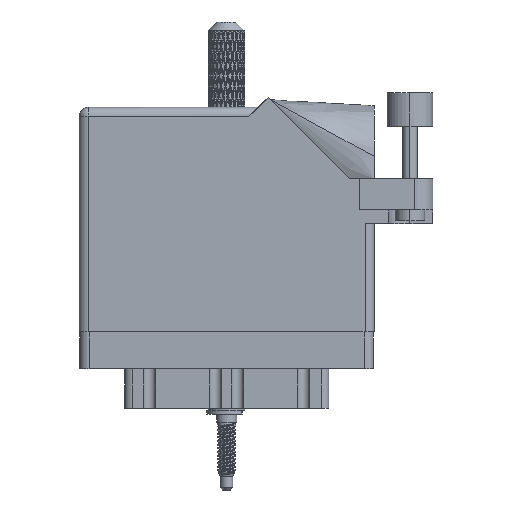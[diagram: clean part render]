
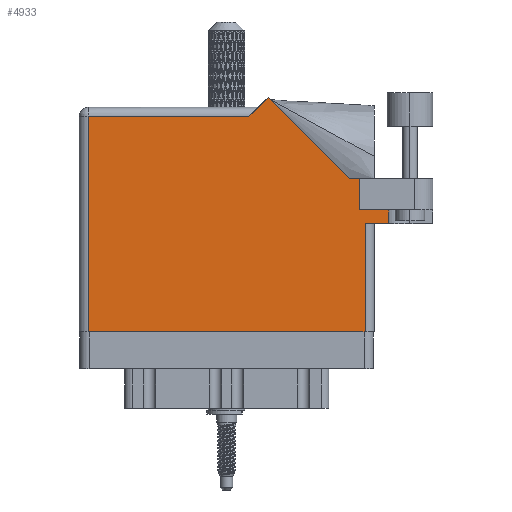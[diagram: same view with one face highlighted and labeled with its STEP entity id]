
A CAD part, front view. The second image highlights one B-rep face of the part: STEP entity #4933.
In plain terms, the highlighted face is planar.
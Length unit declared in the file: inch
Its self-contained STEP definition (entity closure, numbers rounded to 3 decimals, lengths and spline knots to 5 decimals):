
#2073 = CARTESIAN_POINT ( 'NONE',  ( 0., 1.468, 0. ) ) ;
#2655 = VECTOR ( 'NONE', #67782, 39.37008 ) ;
#2757 = CARTESIAN_POINT ( 'NONE',  ( 0.062, 1.468, 0. ) ) ;
#2888 = LINE ( 'NONE', #51669, #55897 ) ;
#3194 = CARTESIAN_POINT ( 'NONE',  ( 1.28771, 1.60071, 0. ) ) ;
#3305 = ORIENTED_EDGE ( 'NONE', *, *, #72947, .T. ) ;
#4055 = DIRECTION ( 'NONE',  ( 1., 0., 0. ) ) ;
#4379 = VECTOR ( 'NONE', #51262, 39.37008 ) ;
#4933 = ADVANCED_FACE ( 'NONE', ( #61687 ), #69104, .F. ) ;
#5165 = ORIENTED_EDGE ( 'NONE', *, *, #74992, .F. ) ;
#5422 = VERTEX_POINT ( 'NONE', #87947 ) ;
#8835 = ORIENTED_EDGE ( 'NONE', *, *, #32671, .F. ) ;
#10510 = EDGE_CURVE ( 'NONE', #98505, #39242, #65467, .T. ) ;
#13570 = CARTESIAN_POINT ( 'NONE',  ( 1.91, 0.831, 0. ) ) ;
#14255 = EDGE_CURVE ( 'NONE', #56066, #93212, #92200, .T. ) ;
#14977 = CARTESIAN_POINT ( 'NONE',  ( 1.948, 0., 0. ) ) ;
#15754 = CARTESIAN_POINT ( 'NONE',  ( 0.062, 0., 0. ) ) ;
#16635 = CARTESIAN_POINT ( 'NONE',  ( 2.1115, 0.831, 0. ) ) ;
#18187 = DIRECTION ( 'NONE',  ( 0., 1., 0. ) ) ;
#18232 = DIRECTION ( 'NONE',  ( 1., 0., 0. ) ) ;
#18774 = ORIENTED_EDGE ( 'NONE', *, *, #67635, .T. ) ;
#19482 = VECTOR ( 'NONE', #30221, 39.37008 ) ;
#20450 = CARTESIAN_POINT ( 'NONE',  ( 2.41, 1.044, 0. ) ) ;
#21317 = VECTOR ( 'NONE', #47770, 39.37008 ) ;
#22718 = ORIENTED_EDGE ( 'NONE', *, *, #14255, .T. ) ;
#23442 = CARTESIAN_POINT ( 'NONE',  ( 1.948, 0.737, 0. ) ) ;
#27198 = LINE ( 'NONE', #104330, #74530 ) ;
#27786 = VERTEX_POINT ( 'NONE', #16635 ) ;
#29893 = VERTEX_POINT ( 'NONE', #14977 ) ;
#30221 = DIRECTION ( 'NONE',  ( -0.707, -0.707, 0. ) ) ;
#32671 = EDGE_CURVE ( 'NONE', #27786, #39242, #2888, .T. ) ;
#33191 = VECTOR ( 'NONE', #87369, 39.37008 ) ;
#38700 = VERTEX_POINT ( 'NONE', #52278 ) ;
#39242 = VERTEX_POINT ( 'NONE', #104354 ) ;
#44265 = DIRECTION ( 'NONE',  ( 0., -1., 0. ) ) ;
#45303 = ORIENTED_EDGE ( 'NONE', *, *, #71131, .T. ) ;
#45427 = DIRECTION ( 'NONE',  ( 1., 0., 0. ) ) ;
#45730 = ORIENTED_EDGE ( 'NONE', *, *, #55389, .T. ) ;
#46623 = VECTOR ( 'NONE', #94030, 39.37008 ) ;
#47770 = DIRECTION ( 'NONE',  ( -0.707, 0.707, 0. ) ) ;
#47938 = EDGE_LOOP ( 'NONE', ( #18774, #45730, #48015, #8835, #5165, #84794, #3305, #103992, #45303, #22718, #99225 ) ) ;
#48015 = ORIENTED_EDGE ( 'NONE', *, *, #10510, .T. ) ;
#51262 = DIRECTION ( 'NONE',  ( -1., 0., 0. ) ) ;
#51669 = CARTESIAN_POINT ( 'NONE',  ( 2.1115, 1.16177, 0. ) ) ;
#52278 = CARTESIAN_POINT ( 'NONE',  ( 1.91, 0.831, 0. ) ) ;
#53980 = AXIS2_PLACEMENT_3D ( 'NONE', #101464, #61173, #63257 ) ;
#54621 = VECTOR ( 'NONE', #18232, 39.37008 ) ;
#55389 = EDGE_CURVE ( 'NONE', #29893, #98505, #63235, .T. ) ;
#55696 = LINE ( 'NONE', #64160, #21317 ) ;
#55897 = VECTOR ( 'NONE', #44265, 39.37008 ) ;
#56066 = VERTEX_POINT ( 'NONE', #85608 ) ;
#57472 = EDGE_CURVE ( 'NONE', #93212, #77820, #88430, .T. ) ;
#59547 = CARTESIAN_POINT ( 'NONE',  ( 1.217, 1.53, 0. ) ) ;
#61173 = DIRECTION ( 'NONE',  ( 0., 0., -1. ) ) ;
#61687 = FACE_OUTER_BOUND ( 'NONE', #47938, .T. ) ;
#63235 = LINE ( 'NONE', #23442, #46623 ) ;
#63257 = DIRECTION ( 'NONE',  ( -1., 0., 0. ) ) ;
#64160 = CARTESIAN_POINT ( 'NONE',  ( 1.84442, 1.044, 0. ) ) ;
#65467 = LINE ( 'NONE', #89890, #54621 ) ;
#67635 = EDGE_CURVE ( 'NONE', #77820, #29893, #68750, .T. ) ;
#67679 = CARTESIAN_POINT ( 'NONE',  ( 1.91, 1.044, 0. ) ) ;
#67782 = DIRECTION ( 'NONE',  ( -1., 0., 0. ) ) ;
#68750 = LINE ( 'NONE', #83107, #70322 ) ;
#69104 = PLANE ( 'NONE',  #53980 ) ;
#70111 = VERTEX_POINT ( 'NONE', #3194 ) ;
#70116 = CARTESIAN_POINT ( 'NONE',  ( 1.948, 0.737, 0. ) ) ;
#70322 = VECTOR ( 'NONE', #4055, 39.37008 ) ;
#71131 = EDGE_CURVE ( 'NONE', #70111, #56066, #100910, .T. ) ;
#72493 = EDGE_CURVE ( 'NONE', #5422, #70111, #55696, .T. ) ;
#72947 = EDGE_CURVE ( 'NONE', #73842, #5422, #73058, .T. ) ;
#73058 = LINE ( 'NONE', #20450, #4379 ) ;
#73842 = VERTEX_POINT ( 'NONE', #67679 ) ;
#74530 = VECTOR ( 'NONE', #18187, 39.37008 ) ;
#74992 = EDGE_CURVE ( 'NONE', #38700, #27786, #101088, .T. ) ;
#77820 = VERTEX_POINT ( 'NONE', #104009 ) ;
#83107 = CARTESIAN_POINT ( 'NONE',  ( 0., 0., 0. ) ) ;
#84771 = EDGE_CURVE ( 'NONE', #38700, #73842, #27198, .T. ) ;
#84794 = ORIENTED_EDGE ( 'NONE', *, *, #84771, .T. ) ;
#85608 = CARTESIAN_POINT ( 'NONE',  ( 1.155, 1.468, 0. ) ) ;
#87369 = DIRECTION ( 'NONE',  ( 0., -1., 0. ) ) ;
#87947 = CARTESIAN_POINT ( 'NONE',  ( 1.84442, 1.044, 0. ) ) ;
#88430 = LINE ( 'NONE', #15754, #33191 ) ;
#89890 = CARTESIAN_POINT ( 'NONE',  ( 2.01, 0.737, 0. ) ) ;
#92200 = LINE ( 'NONE', #2073, #2655 ) ;
#93212 = VERTEX_POINT ( 'NONE', #2757 ) ;
#94030 = DIRECTION ( 'NONE',  ( 0., 1., 0. ) ) ;
#98505 = VERTEX_POINT ( 'NONE', #70116 ) ;
#99225 = ORIENTED_EDGE ( 'NONE', *, *, #57472, .T. ) ;
#100910 = LINE ( 'NONE', #59547, #19482 ) ;
#101052 = VECTOR ( 'NONE', #45427, 39.37008 ) ;
#101088 = LINE ( 'NONE', #13570, #101052 ) ;
#101464 = CARTESIAN_POINT ( 'NONE',  ( 0., 1.53, 0. ) ) ;
#103992 = ORIENTED_EDGE ( 'NONE', *, *, #72493, .T. ) ;
#104009 = CARTESIAN_POINT ( 'NONE',  ( 0.062, 0., 0. ) ) ;
#104330 = CARTESIAN_POINT ( 'NONE',  ( 1.91, 0.831, 0. ) ) ;
#104354 = CARTESIAN_POINT ( 'NONE',  ( 2.1115, 0.737, 0. ) ) ;
